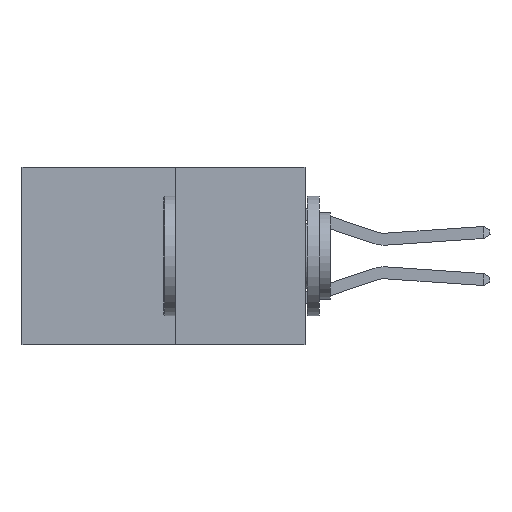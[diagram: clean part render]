
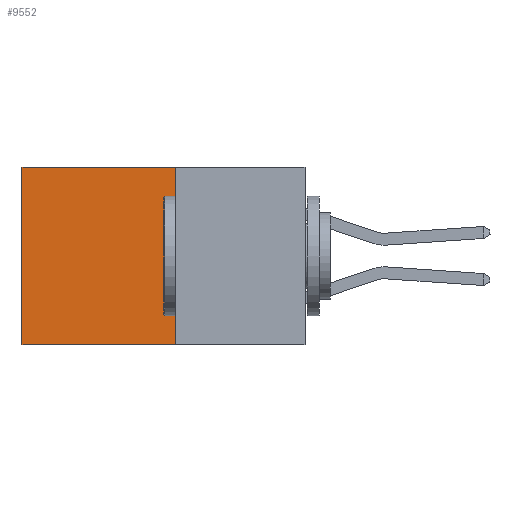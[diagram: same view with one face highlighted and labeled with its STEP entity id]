
A CAD part, left-side view. The second image highlights one B-rep face of the part: STEP entity #9552.
In plain terms, the highlighted planar face has unit normal (-1, 0, 0).
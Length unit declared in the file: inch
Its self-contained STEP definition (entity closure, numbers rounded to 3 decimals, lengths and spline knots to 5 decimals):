
#209 = CARTESIAN_POINT ( 'NONE',  ( 0.277, 0.59, 0. ) ) ;
#219 = ORIENTED_EDGE ( 'NONE', *, *, #2277, .F. ) ;
#284 = AXIS2_PLACEMENT_3D ( 'NONE', #1840, #9030, #2961 ) ;
#920 = LINE ( 'NONE', #9300, #6103 ) ;
#1356 = VERTEX_POINT ( 'NONE', #3171 ) ;
#1840 = CARTESIAN_POINT ( 'NONE',  ( 0.277, 0.27, -0.37 ) ) ;
#2117 = FACE_OUTER_BOUND ( 'NONE', #9895, .T. ) ;
#2277 = EDGE_CURVE ( 'NONE', #9253, #1356, #8521, .T. ) ;
#2961 = DIRECTION ( 'NONE',  ( 0., 0., -1. ) ) ;
#3171 = CARTESIAN_POINT ( 'NONE',  ( 0.277, 0.27, -0.37 ) ) ;
#3829 = CARTESIAN_POINT ( 'NONE',  ( 0.277, 0.59, -0.37 ) ) ;
#3888 = ORIENTED_EDGE ( 'NONE', *, *, #13240, .T. ) ;
#4003 = VERTEX_POINT ( 'NONE', #209 ) ;
#4310 = EDGE_CURVE ( 'NONE', #1356, #12921, #10057, .T. ) ;
#4829 = DIRECTION ( 'NONE',  ( 0., 1., 0. ) ) ;
#5011 = ORIENTED_EDGE ( 'NONE', *, *, #4310, .F. ) ;
#5062 = DIRECTION ( 'NONE',  ( 0., 0., -1. ) ) ;
#5826 = VECTOR ( 'NONE', #5062, 39.37008 ) ;
#6103 = VECTOR ( 'NONE', #10290, 39.37008 ) ;
#6333 = CARTESIAN_POINT ( 'NONE',  ( 0.277, 0.27, 0. ) ) ;
#6971 = PLANE ( 'NONE',  #284 ) ;
#6997 = VECTOR ( 'NONE', #9409, 39.37008 ) ;
#7329 = LINE ( 'NONE', #6333, #6997 ) ;
#7951 = CARTESIAN_POINT ( 'NONE',  ( 0.277, 0.27, -0.37 ) ) ;
#8164 = ORIENTED_EDGE ( 'NONE', *, *, #12002, .T. ) ;
#8521 = LINE ( 'NONE', #12658, #5826 ) ;
#9030 = DIRECTION ( 'NONE',  ( 1., 0., 0. ) ) ;
#9253 = VERTEX_POINT ( 'NONE', #9529 ) ;
#9300 = CARTESIAN_POINT ( 'NONE',  ( 0.277, 0.59, -0.37 ) ) ;
#9409 = DIRECTION ( 'NONE',  ( 0., 1., 0. ) ) ;
#9529 = CARTESIAN_POINT ( 'NONE',  ( 0.277, 0.27, 0. ) ) ;
#9552 = ADVANCED_FACE ( 'NONE', ( #2117 ), #6971, .F. ) ;
#9895 = EDGE_LOOP ( 'NONE', ( #8164, #5011, #219, #3888 ) ) ;
#10057 = LINE ( 'NONE', #7951, #12466 ) ;
#10290 = DIRECTION ( 'NONE',  ( 0., 0., -1. ) ) ;
#12002 = EDGE_CURVE ( 'NONE', #4003, #12921, #920, .T. ) ;
#12466 = VECTOR ( 'NONE', #4829, 39.37008 ) ;
#12658 = CARTESIAN_POINT ( 'NONE',  ( 0.277, 0.27, -0.37 ) ) ;
#12921 = VERTEX_POINT ( 'NONE', #3829 ) ;
#13240 = EDGE_CURVE ( 'NONE', #9253, #4003, #7329, .T. ) ;
